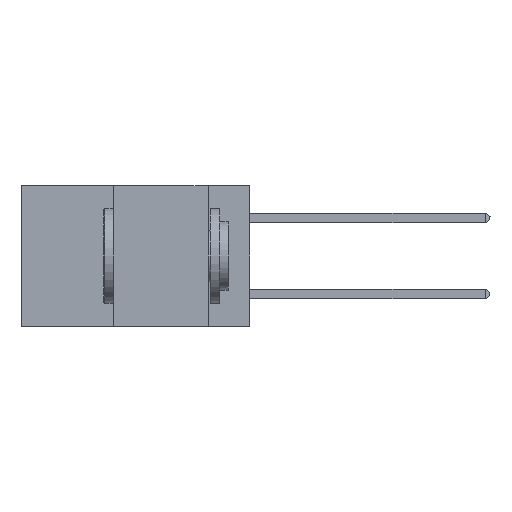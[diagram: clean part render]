
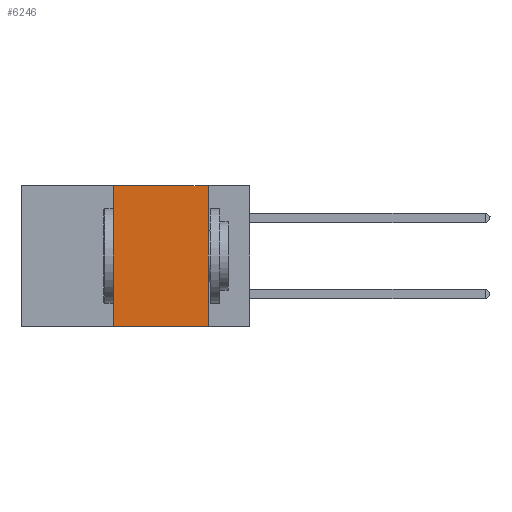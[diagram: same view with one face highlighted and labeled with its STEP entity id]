
A CAD part, left-side view. The second image highlights one B-rep face of the part: STEP entity #6246.
In plain terms, the highlighted planar face has unit normal (-1, 0, 0).
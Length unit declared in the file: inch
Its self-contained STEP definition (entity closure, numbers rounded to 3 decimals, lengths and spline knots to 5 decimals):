
#840 = LINE ( 'NONE', #8834, #17438 ) ;
#1477 = EDGE_CURVE ( 'NONE', #16279, #13218, #6355, .T. ) ;
#2344 = CARTESIAN_POINT ( 'NONE',  ( 0., 0.36, 0. ) ) ;
#2456 = LINE ( 'NONE', #17788, #6829 ) ;
#3090 = AXIS2_PLACEMENT_3D ( 'NONE', #14606, #5051, #16142 ) ;
#3340 = CARTESIAN_POINT ( 'NONE',  ( 0., 0.11, 0. ) ) ;
#5051 = DIRECTION ( 'NONE',  ( 1., 0., 0. ) ) ;
#5108 = VERTEX_POINT ( 'NONE', #3340 ) ;
#5510 = EDGE_CURVE ( 'NONE', #5108, #13218, #2456, .T. ) ;
#6246 = ADVANCED_FACE ( 'NONE', ( #9838 ), #11502, .F. ) ;
#6355 = LINE ( 'NONE', #7504, #9125 ) ;
#6829 = VECTOR ( 'NONE', #19318, 39.37008 ) ;
#7392 = DIRECTION ( 'NONE',  ( 0., -1., 0. ) ) ;
#7504 = CARTESIAN_POINT ( 'NONE',  ( 0., 0.6, -0.37 ) ) ;
#8508 = DIRECTION ( 'NONE',  ( 0., -1., 0. ) ) ;
#8834 = CARTESIAN_POINT ( 'NONE',  ( 0., 0.36, 0. ) ) ;
#9125 = VECTOR ( 'NONE', #7392, 39.37008 ) ;
#9838 = FACE_OUTER_BOUND ( 'NONE', #18886, .T. ) ;
#10231 = CARTESIAN_POINT ( 'NONE',  ( 0., 0.11, -0.37 ) ) ;
#10591 = EDGE_CURVE ( 'NONE', #19491, #5108, #13136, .T. ) ;
#11502 = PLANE ( 'NONE',  #3090 ) ;
#11600 = ORIENTED_EDGE ( 'NONE', *, *, #19532, .F. ) ;
#13136 = LINE ( 'NONE', #13286, #16747 ) ;
#13218 = VERTEX_POINT ( 'NONE', #10231 ) ;
#13286 = CARTESIAN_POINT ( 'NONE',  ( 0., 0.6, 0. ) ) ;
#13703 = DIRECTION ( 'NONE',  ( 0., 0., 1. ) ) ;
#13741 = CARTESIAN_POINT ( 'NONE',  ( 0., 0.36, -0.37 ) ) ;
#14606 = CARTESIAN_POINT ( 'NONE',  ( 0., 0.6, 0. ) ) ;
#16142 = DIRECTION ( 'NONE',  ( 0., 0., -1. ) ) ;
#16279 = VERTEX_POINT ( 'NONE', #13741 ) ;
#16747 = VECTOR ( 'NONE', #8508, 39.37008 ) ;
#17438 = VECTOR ( 'NONE', #13703, 39.37008 ) ;
#17788 = CARTESIAN_POINT ( 'NONE',  ( 0., 0.11, 0. ) ) ;
#18243 = ORIENTED_EDGE ( 'NONE', *, *, #5510, .F. ) ;
#18869 = ORIENTED_EDGE ( 'NONE', *, *, #10591, .F. ) ;
#18886 = EDGE_LOOP ( 'NONE', ( #18243, #18869, #11600, #19088 ) ) ;
#19088 = ORIENTED_EDGE ( 'NONE', *, *, #1477, .T. ) ;
#19318 = DIRECTION ( 'NONE',  ( 0., 0., -1. ) ) ;
#19491 = VERTEX_POINT ( 'NONE', #2344 ) ;
#19532 = EDGE_CURVE ( 'NONE', #16279, #19491, #840, .T. ) ;
